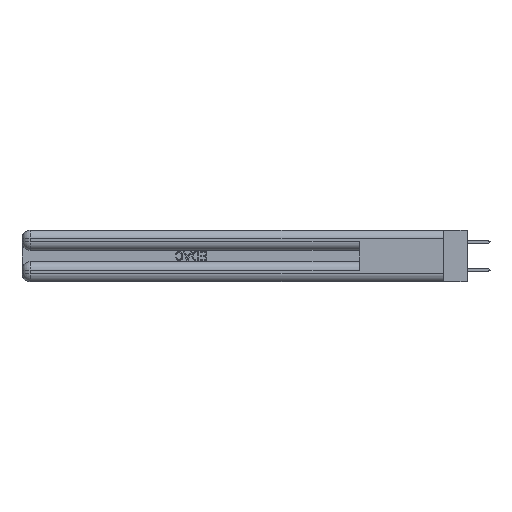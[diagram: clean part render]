
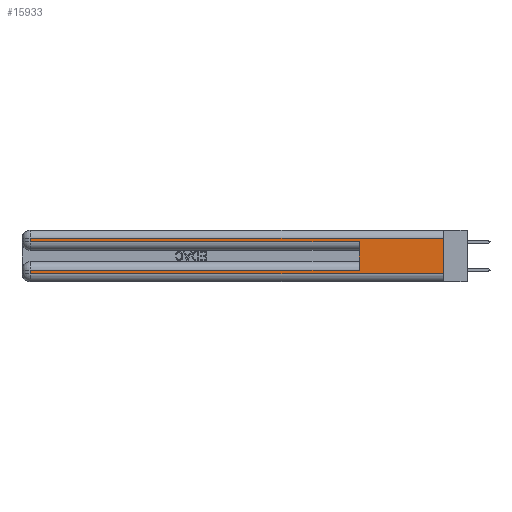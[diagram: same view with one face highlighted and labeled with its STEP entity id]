
A CAD part, left-side view. The second image highlights one B-rep face of the part: STEP entity #15933.
In plain terms, the highlighted planar face has unit normal (-1, 0, 0).
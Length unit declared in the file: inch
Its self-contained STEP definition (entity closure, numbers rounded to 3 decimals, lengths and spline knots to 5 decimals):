
#868 = VECTOR ( 'NONE', #17291, 39.37008 ) ;
#2663 = CARTESIAN_POINT ( 'NONE',  ( 0., 0., 0.285 ) ) ;
#3061 = LINE ( 'NONE', #8436, #27703 ) ;
#3483 = CARTESIAN_POINT ( 'NONE',  ( 0., 2.94, 0.31 ) ) ;
#3624 = VERTEX_POINT ( 'NONE', #3483 ) ;
#5772 = VECTOR ( 'NONE', #32157, 39.37008 ) ;
#7533 = ORIENTED_EDGE ( 'NONE', *, *, #9642, .T. ) ;
#7804 = EDGE_CURVE ( 'NONE', #11195, #17015, #3061, .T. ) ;
#8436 = CARTESIAN_POINT ( 'NONE',  ( 0., 0., 0.06 ) ) ;
#8556 = LINE ( 'NONE', #2663, #17114 ) ;
#9106 = CARTESIAN_POINT ( 'NONE',  ( 0., 0.6, 0.285 ) ) ;
#9642 = EDGE_CURVE ( 'NONE', #21037, #20644, #26534, .T. ) ;
#9674 = CARTESIAN_POINT ( 'NONE',  ( 0., 0., 0.31 ) ) ;
#9953 = VERTEX_POINT ( 'NONE', #9106 ) ;
#10241 = ORIENTED_EDGE ( 'NONE', *, *, #20099, .T. ) ;
#10249 = CARTESIAN_POINT ( 'NONE',  ( 0., 2.94, 0.06 ) ) ;
#11195 = VERTEX_POINT ( 'NONE', #10249 ) ;
#11543 = CARTESIAN_POINT ( 'NONE',  ( 0., 0.6, 0.085 ) ) ;
#11810 = EDGE_CURVE ( 'NONE', #20644, #11195, #30384, .T. ) ;
#13024 = CARTESIAN_POINT ( 'NONE',  ( 0., 2.94, 0.37 ) ) ;
#13131 = DIRECTION ( 'NONE',  ( 0., 0., 1. ) ) ;
#14229 = EDGE_CURVE ( 'NONE', #20209, #17015, #20147, .T. ) ;
#15933 = ADVANCED_FACE ( 'NONE', ( #17066 ), #32403, .F. ) ;
#16098 = DIRECTION ( 'NONE',  ( 0., 0., -1. ) ) ;
#16398 = CARTESIAN_POINT ( 'NONE',  ( 0., 0., 0.37 ) ) ;
#17015 = VERTEX_POINT ( 'NONE', #36301 ) ;
#17066 = FACE_OUTER_BOUND ( 'NONE', #35323, .T. ) ;
#17114 = VECTOR ( 'NONE', #25170, 39.37008 ) ;
#17291 = DIRECTION ( 'NONE',  ( 0., 1., 0. ) ) ;
#17889 = ORIENTED_EDGE ( 'NONE', *, *, #14229, .F. ) ;
#18106 = DIRECTION ( 'NONE',  ( 0., -1., 0. ) ) ;
#19609 = DIRECTION ( 'NONE',  ( 0., 0., -1. ) ) ;
#20099 = EDGE_CURVE ( 'NONE', #3624, #22900, #28256, .T. ) ;
#20147 = LINE ( 'NONE', #32803, #35222 ) ;
#20209 = VERTEX_POINT ( 'NONE', #26317 ) ;
#20644 = VERTEX_POINT ( 'NONE', #22248 ) ;
#20715 = EDGE_CURVE ( 'NONE', #21037, #9953, #27280, .T. ) ;
#21037 = VERTEX_POINT ( 'NONE', #11543 ) ;
#21048 = ORIENTED_EDGE ( 'NONE', *, *, #7804, .T. ) ;
#21914 = ORIENTED_EDGE ( 'NONE', *, *, #11810, .T. ) ;
#22248 = CARTESIAN_POINT ( 'NONE',  ( 0., 2.94, 0.085 ) ) ;
#22900 = VERTEX_POINT ( 'NONE', #30403 ) ;
#25170 = DIRECTION ( 'NONE',  ( 0., -1., 0. ) ) ;
#26317 = CARTESIAN_POINT ( 'NONE',  ( 0., 0., 0.31 ) ) ;
#26534 = LINE ( 'NONE', #36519, #868 ) ;
#27280 = LINE ( 'NONE', #35423, #33811 ) ;
#27703 = VECTOR ( 'NONE', #18106, 39.37008 ) ;
#28256 = LINE ( 'NONE', #13024, #36804 ) ;
#29368 = VECTOR ( 'NONE', #32826, 39.37008 ) ;
#29586 = DIRECTION ( 'NONE',  ( 0., 0., -1. ) ) ;
#29827 = EDGE_CURVE ( 'NONE', #20209, #3624, #30410, .T. ) ;
#30384 = LINE ( 'NONE', #36052, #29368 ) ;
#30403 = CARTESIAN_POINT ( 'NONE',  ( 0., 2.94, 0.285 ) ) ;
#30410 = LINE ( 'NONE', #9674, #5772 ) ;
#32157 = DIRECTION ( 'NONE',  ( 0., 1., 0. ) ) ;
#32403 = PLANE ( 'NONE',  #36557 ) ;
#32602 = ORIENTED_EDGE ( 'NONE', *, *, #20715, .F. ) ;
#32803 = CARTESIAN_POINT ( 'NONE',  ( 0., 0., 0.37 ) ) ;
#32826 = DIRECTION ( 'NONE',  ( 0., 0., -1. ) ) ;
#33811 = VECTOR ( 'NONE', #13131, 39.37008 ) ;
#34029 = ORIENTED_EDGE ( 'NONE', *, *, #38421, .T. ) ;
#35222 = VECTOR ( 'NONE', #29586, 39.37008 ) ;
#35323 = EDGE_LOOP ( 'NONE', ( #17889, #36687, #10241, #34029, #32602, #7533, #21914, #21048 ) ) ;
#35423 = CARTESIAN_POINT ( 'NONE',  ( 0., 0.6, 0.145 ) ) ;
#36052 = CARTESIAN_POINT ( 'NONE',  ( 0., 2.94, 0.37 ) ) ;
#36301 = CARTESIAN_POINT ( 'NONE',  ( 0., 0., 0.06 ) ) ;
#36519 = CARTESIAN_POINT ( 'NONE',  ( 0., 0., 0.085 ) ) ;
#36557 = AXIS2_PLACEMENT_3D ( 'NONE', #16398, #38839, #19609 ) ;
#36687 = ORIENTED_EDGE ( 'NONE', *, *, #29827, .T. ) ;
#36804 = VECTOR ( 'NONE', #16098, 39.37008 ) ;
#38421 = EDGE_CURVE ( 'NONE', #22900, #9953, #8556, .T. ) ;
#38839 = DIRECTION ( 'NONE',  ( 1., 0., 0. ) ) ;
